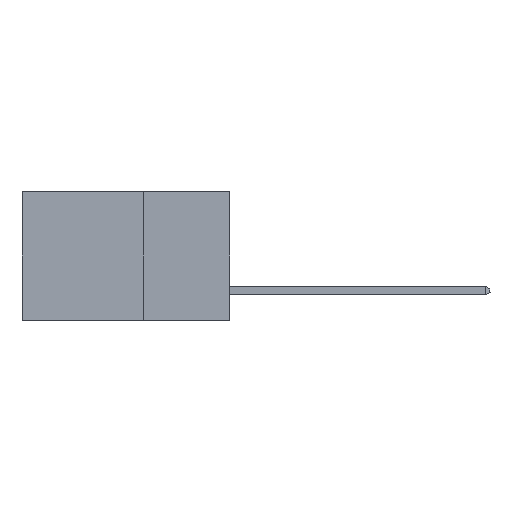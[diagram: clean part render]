
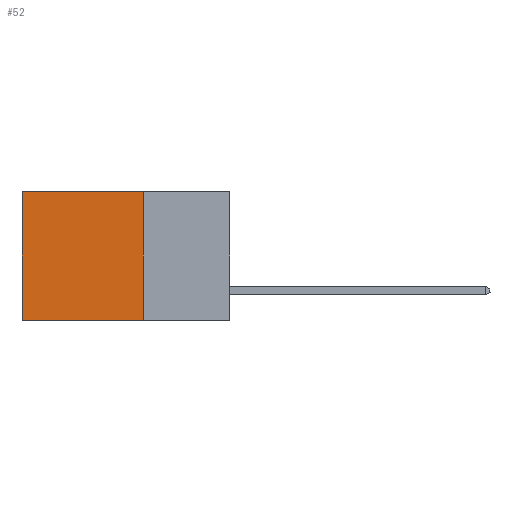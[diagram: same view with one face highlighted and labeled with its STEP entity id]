
A CAD part, left-side view. The second image highlights one B-rep face of the part: STEP entity #52.
In plain terms, the highlighted planar face has unit normal (-1, 0, 0).
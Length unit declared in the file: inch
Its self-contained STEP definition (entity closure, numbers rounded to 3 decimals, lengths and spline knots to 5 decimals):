
#52 = ADVANCED_FACE ( 'NONE', ( #10731 ), #9095, .F. ) ;
#540 = DIRECTION ( 'NONE',  ( 0., 0., -1. ) ) ;
#575 = VECTOR ( 'NONE', #1411, 39.37008 ) ;
#657 = ORIENTED_EDGE ( 'NONE', *, *, #9121, .F. ) ;
#1411 = DIRECTION ( 'NONE',  ( 0., 0., -1. ) ) ;
#1606 = ORIENTED_EDGE ( 'NONE', *, *, #6329, .T. ) ;
#1699 = LINE ( 'NONE', #4655, #6505 ) ;
#2181 = CARTESIAN_POINT ( 'NONE',  ( 0.298, 0.6, -0.37 ) ) ;
#2234 = CARTESIAN_POINT ( 'NONE',  ( 0.298, 0.6, 0. ) ) ;
#3011 = DIRECTION ( 'NONE',  ( 1., 0., 0. ) ) ;
#3123 = EDGE_CURVE ( 'NONE', #4261, #9330, #4685, .T. ) ;
#3478 = LINE ( 'NONE', #2234, #575 ) ;
#3487 = VECTOR ( 'NONE', #10925, 39.37008 ) ;
#3891 = EDGE_CURVE ( 'NONE', #7320, #10500, #3478, .T. ) ;
#3949 = ORIENTED_EDGE ( 'NONE', *, *, #3123, .F. ) ;
#4261 = VERTEX_POINT ( 'NONE', #5277 ) ;
#4655 = CARTESIAN_POINT ( 'NONE',  ( 0.298, 0.25, 0. ) ) ;
#4685 = LINE ( 'NONE', #9848, #5372 ) ;
#4711 = ORIENTED_EDGE ( 'NONE', *, *, #3891, .T. ) ;
#5277 = CARTESIAN_POINT ( 'NONE',  ( 0.298, 0.25, 0. ) ) ;
#5372 = VECTOR ( 'NONE', #540, 39.37008 ) ;
#5774 = LINE ( 'NONE', #9177, #3487 ) ;
#6211 = CARTESIAN_POINT ( 'NONE',  ( 0.298, 0.25, -0.37 ) ) ;
#6329 = EDGE_CURVE ( 'NONE', #4261, #7320, #1699, .T. ) ;
#6404 = AXIS2_PLACEMENT_3D ( 'NONE', #7268, #3011, #8950 ) ;
#6505 = VECTOR ( 'NONE', #10573, 39.37008 ) ;
#7268 = CARTESIAN_POINT ( 'NONE',  ( 0.298, 0.25, 0. ) ) ;
#7320 = VERTEX_POINT ( 'NONE', #7973 ) ;
#7973 = CARTESIAN_POINT ( 'NONE',  ( 0.298, 0.6, 0. ) ) ;
#8809 = EDGE_LOOP ( 'NONE', ( #4711, #657, #3949, #1606 ) ) ;
#8950 = DIRECTION ( 'NONE',  ( 0., 0., -1. ) ) ;
#9095 = PLANE ( 'NONE',  #6404 ) ;
#9121 = EDGE_CURVE ( 'NONE', #9330, #10500, #5774, .T. ) ;
#9177 = CARTESIAN_POINT ( 'NONE',  ( 0.298, 0.25, -0.37 ) ) ;
#9330 = VERTEX_POINT ( 'NONE', #6211 ) ;
#9848 = CARTESIAN_POINT ( 'NONE',  ( 0.298, 0.25, 0. ) ) ;
#10500 = VERTEX_POINT ( 'NONE', #2181 ) ;
#10573 = DIRECTION ( 'NONE',  ( 0., 1., 0. ) ) ;
#10731 = FACE_OUTER_BOUND ( 'NONE', #8809, .T. ) ;
#10925 = DIRECTION ( 'NONE',  ( 0., 1., 0. ) ) ;
